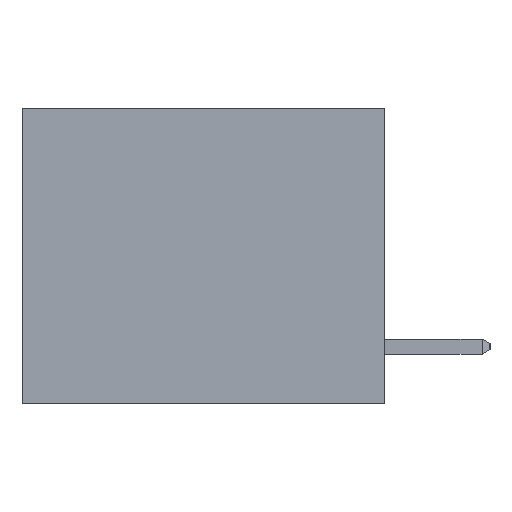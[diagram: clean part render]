
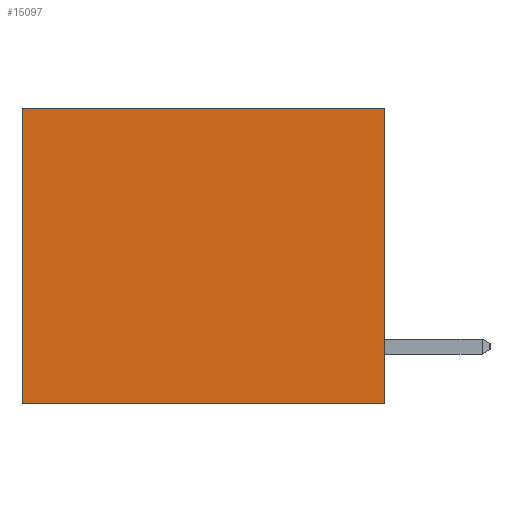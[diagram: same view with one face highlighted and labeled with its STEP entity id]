
A CAD part, left-side view. The second image highlights one B-rep face of the part: STEP entity #15097.
In plain terms, the highlighted planar face has unit normal (-1, 0, 0).
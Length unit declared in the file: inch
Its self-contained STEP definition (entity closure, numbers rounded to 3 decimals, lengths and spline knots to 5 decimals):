
#432 = CARTESIAN_POINT ( 'NONE',  ( 0.3165, 0., 0. ) ) ;
#3298 = ORIENTED_EDGE ( 'NONE', *, *, #14855, .T. ) ;
#3635 = DIRECTION ( 'NONE',  ( 0., 0., -1. ) ) ;
#3676 = DIRECTION ( 'NONE',  ( 0., 1., 0. ) ) ;
#4072 = VECTOR ( 'NONE', #19093, 39.37008 ) ;
#4526 = VERTEX_POINT ( 'NONE', #16343 ) ;
#5848 = LINE ( 'NONE', #9986, #21473 ) ;
#6815 = EDGE_CURVE ( 'NONE', #17011, #4526, #8502, .T. ) ;
#7186 = DIRECTION ( 'NONE',  ( 1., 0., 0. ) ) ;
#8060 = VERTEX_POINT ( 'NONE', #432 ) ;
#8502 = LINE ( 'NONE', #24212, #15807 ) ;
#9986 = CARTESIAN_POINT ( 'NONE',  ( 0.3165, 0., 0. ) ) ;
#10195 = CARTESIAN_POINT ( 'NONE',  ( 0.3165, 0., -0.49 ) ) ;
#12101 = AXIS2_PLACEMENT_3D ( 'NONE', #15837, #7186, #24727 ) ;
#12448 = CARTESIAN_POINT ( 'NONE',  ( 0.3165, 0.6, -0.49 ) ) ;
#14386 = ORIENTED_EDGE ( 'NONE', *, *, #6815, .F. ) ;
#14855 = EDGE_CURVE ( 'NONE', #25079, #4526, #27934, .T. ) ;
#15097 = ADVANCED_FACE ( 'NONE', ( #23052 ), #22518, .F. ) ;
#15807 = VECTOR ( 'NONE', #26157, 39.37008 ) ;
#15837 = CARTESIAN_POINT ( 'NONE',  ( 0.3165, 0., -0.49 ) ) ;
#15902 = LINE ( 'NONE', #10195, #4072 ) ;
#16266 = ORIENTED_EDGE ( 'NONE', *, *, #27443, .F. ) ;
#16343 = CARTESIAN_POINT ( 'NONE',  ( 0.3165, 0.6, -0.49 ) ) ;
#16531 = EDGE_LOOP ( 'NONE', ( #3298, #14386, #16266, #23212 ) ) ;
#17011 = VERTEX_POINT ( 'NONE', #24627 ) ;
#18119 = EDGE_CURVE ( 'NONE', #8060, #25079, #5848, .T. ) ;
#19093 = DIRECTION ( 'NONE',  ( 0., 0., -1. ) ) ;
#21473 = VECTOR ( 'NONE', #3676, 39.37008 ) ;
#22518 = PLANE ( 'NONE',  #12101 ) ;
#23052 = FACE_OUTER_BOUND ( 'NONE', #16531, .T. ) ;
#23078 = VECTOR ( 'NONE', #3635, 39.37008 ) ;
#23212 = ORIENTED_EDGE ( 'NONE', *, *, #18119, .T. ) ;
#24212 = CARTESIAN_POINT ( 'NONE',  ( 0.3165, 0., -0.49 ) ) ;
#24627 = CARTESIAN_POINT ( 'NONE',  ( 0.3165, 0., -0.49 ) ) ;
#24727 = DIRECTION ( 'NONE',  ( 0., 0., -1. ) ) ;
#25079 = VERTEX_POINT ( 'NONE', #28239 ) ;
#26157 = DIRECTION ( 'NONE',  ( 0., 1., 0. ) ) ;
#27443 = EDGE_CURVE ( 'NONE', #8060, #17011, #15902, .T. ) ;
#27934 = LINE ( 'NONE', #12448, #23078 ) ;
#28239 = CARTESIAN_POINT ( 'NONE',  ( 0.3165, 0.6, 0. ) ) ;
